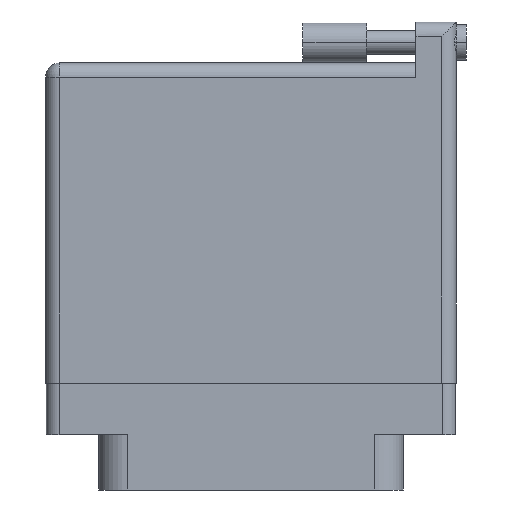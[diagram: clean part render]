
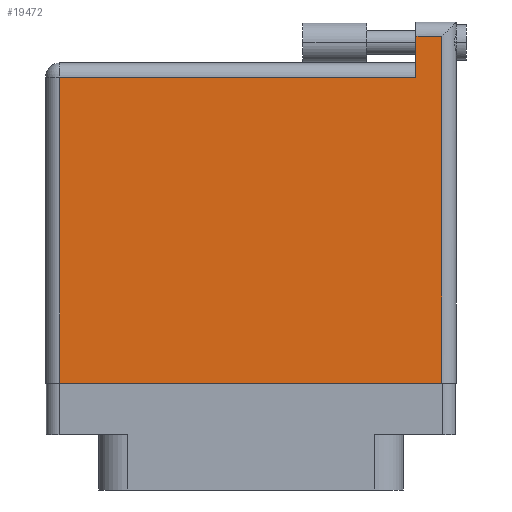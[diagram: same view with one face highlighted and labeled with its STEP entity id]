
A CAD part, front view. The second image highlights one B-rep face of the part: STEP entity #19472.
In plain terms, the highlighted face is planar.
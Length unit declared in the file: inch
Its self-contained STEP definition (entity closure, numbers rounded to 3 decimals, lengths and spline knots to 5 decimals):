
#367 = CARTESIAN_POINT ( 'NONE',  ( -1.004, -0.1, 0.4495 ) ) ;
#824 = LINE ( 'NONE', #31137, #17295 ) ;
#1279 = CARTESIAN_POINT ( 'NONE',  ( -1.004, 1.396, 0.4495 ) ) ;
#2002 = VECTOR ( 'NONE', #12627, 39.37008 ) ;
#3084 = PLANE ( 'NONE',  #36991 ) ;
#3467 = ORIENTED_EDGE ( 'NONE', *, *, #18622, .T. ) ;
#3809 = EDGE_CURVE ( 'NONE', #5289, #10792, #37681, .T. ) ;
#3946 = CARTESIAN_POINT ( 'NONE',  ( 0.934, 1.666, 0.4495 ) ) ;
#5289 = VERTEX_POINT ( 'NONE', #27020 ) ;
#6518 = CARTESIAN_POINT ( 'NONE',  ( -1.004, 1.466, 0.4495 ) ) ;
#8385 = CARTESIAN_POINT ( 'NONE',  ( -0.934, -0.1, 0.4495 ) ) ;
#9369 = EDGE_CURVE ( 'NONE', #39721, #5289, #18902, .T. ) ;
#9980 = LINE ( 'NONE', #3946, #39520 ) ;
#9997 = CARTESIAN_POINT ( 'NONE',  ( 0.807, 1.666, 0.4495 ) ) ;
#10330 = DIRECTION ( 'NONE',  ( -1., 0., 0. ) ) ;
#10653 = ORIENTED_EDGE ( 'NONE', *, *, #33609, .T. ) ;
#10792 = VERTEX_POINT ( 'NONE', #10920 ) ;
#10920 = CARTESIAN_POINT ( 'NONE',  ( 0.807, 1.396, 0.4495 ) ) ;
#10982 = DIRECTION ( 'NONE',  ( -1., 0., 0. ) ) ;
#11178 = CARTESIAN_POINT ( 'NONE',  ( -1.004, 1.596, 0.4495 ) ) ;
#12627 = DIRECTION ( 'NONE',  ( 0., -1., 0. ) ) ;
#12639 = DIRECTION ( 'NONE',  ( 1., 0., 0. ) ) ;
#13842 = EDGE_CURVE ( 'NONE', #22794, #28157, #27613, .T. ) ;
#14758 = ORIENTED_EDGE ( 'NONE', *, *, #13842, .T. ) ;
#15529 = VERTEX_POINT ( 'NONE', #38639 ) ;
#17295 = VECTOR ( 'NONE', #37157, 39.37008 ) ;
#17779 = VECTOR ( 'NONE', #12639, 39.37008 ) ;
#18622 = EDGE_CURVE ( 'NONE', #28157, #39721, #9980, .T. ) ;
#18830 = DIRECTION ( 'NONE',  ( 0., 0., -1. ) ) ;
#18902 = LINE ( 'NONE', #11178, #20110 ) ;
#19472 = ADVANCED_FACE ( 'NONE', ( #34193 ), #3084, .F. ) ;
#20110 = VECTOR ( 'NONE', #10982, 39.37008 ) ;
#22309 = CARTESIAN_POINT ( 'NONE',  ( 0.934, 1.596, 0.4495 ) ) ;
#22794 = VERTEX_POINT ( 'NONE', #8385 ) ;
#23535 = ORIENTED_EDGE ( 'NONE', *, *, #3809, .T. ) ;
#24643 = EDGE_LOOP ( 'NONE', ( #14758, #3467, #29714, #23535, #31053, #10653 ) ) ;
#27020 = CARTESIAN_POINT ( 'NONE',  ( 0.807, 1.596, 0.4495 ) ) ;
#27613 = LINE ( 'NONE', #367, #17779 ) ;
#28157 = VERTEX_POINT ( 'NONE', #34134 ) ;
#29714 = ORIENTED_EDGE ( 'NONE', *, *, #9369, .T. ) ;
#30582 = DIRECTION ( 'NONE',  ( -1., 0., 0. ) ) ;
#31053 = ORIENTED_EDGE ( 'NONE', *, *, #31597, .T. ) ;
#31137 = CARTESIAN_POINT ( 'NONE',  ( -0.934, -0.1, 0.4495 ) ) ;
#31418 = VECTOR ( 'NONE', #10330, 39.37008 ) ;
#31597 = EDGE_CURVE ( 'NONE', #10792, #15529, #38965, .T. ) ;
#33609 = EDGE_CURVE ( 'NONE', #15529, #22794, #824, .T. ) ;
#34134 = CARTESIAN_POINT ( 'NONE',  ( 0.934, -0.1, 0.4495 ) ) ;
#34193 = FACE_OUTER_BOUND ( 'NONE', #24643, .T. ) ;
#36991 = AXIS2_PLACEMENT_3D ( 'NONE', #6518, #18830, #30582 ) ;
#37157 = DIRECTION ( 'NONE',  ( 0., -1., 0. ) ) ;
#37681 = LINE ( 'NONE', #9997, #2002 ) ;
#38055 = DIRECTION ( 'NONE',  ( 0., 1., 0. ) ) ;
#38639 = CARTESIAN_POINT ( 'NONE',  ( -0.934, 1.396, 0.4495 ) ) ;
#38965 = LINE ( 'NONE', #1279, #31418 ) ;
#39520 = VECTOR ( 'NONE', #38055, 39.37008 ) ;
#39721 = VERTEX_POINT ( 'NONE', #22309 ) ;
